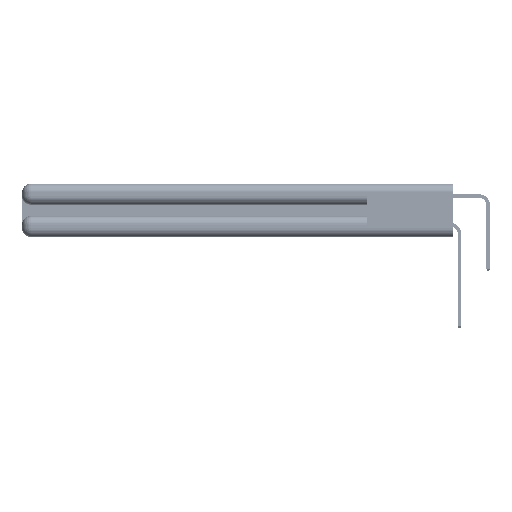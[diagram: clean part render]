
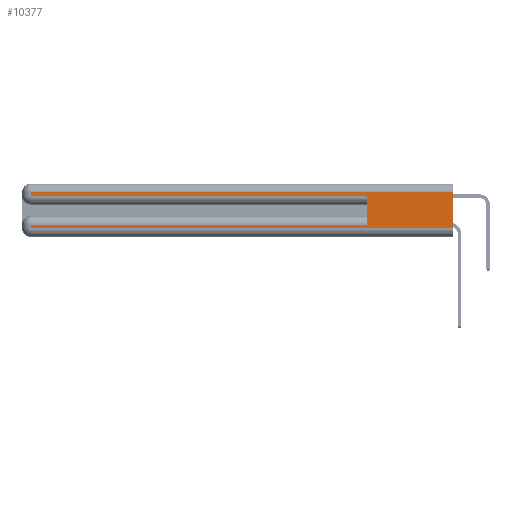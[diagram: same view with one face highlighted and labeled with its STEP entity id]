
A CAD part, left-side view. The second image highlights one B-rep face of the part: STEP entity #10377.
In plain terms, the highlighted planar face has unit normal (-1, 0, 0).
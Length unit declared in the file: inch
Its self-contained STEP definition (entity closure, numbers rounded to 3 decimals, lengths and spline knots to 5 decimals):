
#197 = CARTESIAN_POINT ( 'NONE',  ( 0., 0., 0.37 ) ) ;
#568 = DIRECTION ( 'NONE',  ( 1., 0., 0. ) ) ;
#743 = VECTOR ( 'NONE', #23854, 39.37008 ) ;
#811 = CARTESIAN_POINT ( 'NONE',  ( 0., 0.6, 0.085 ) ) ;
#1697 = ORIENTED_EDGE ( 'NONE', *, *, #26742, .T. ) ;
#2067 = CARTESIAN_POINT ( 'NONE',  ( 0., 0., 0.06 ) ) ;
#2609 = CARTESIAN_POINT ( 'NONE',  ( 0., 2.94, 0.06 ) ) ;
#2709 = LINE ( 'NONE', #13319, #29796 ) ;
#3090 = CARTESIAN_POINT ( 'NONE',  ( 0., 2.94, 0.285 ) ) ;
#3481 = EDGE_CURVE ( 'NONE', #26933, #31815, #48460, .T. ) ;
#3754 = DIRECTION ( 'NONE',  ( 0., 0., -1. ) ) ;
#5217 = VERTEX_POINT ( 'NONE', #19305 ) ;
#6022 = VERTEX_POINT ( 'NONE', #3090 ) ;
#6472 = VECTOR ( 'NONE', #3754, 39.37008 ) ;
#6734 = LINE ( 'NONE', #32748, #34508 ) ;
#7113 = LINE ( 'NONE', #20582, #6472 ) ;
#9104 = CARTESIAN_POINT ( 'NONE',  ( 0., 0., 0.37 ) ) ;
#10043 = LINE ( 'NONE', #11461, #743 ) ;
#10377 = ADVANCED_FACE ( 'NONE', ( #46119 ), #21132, .F. ) ;
#10402 = ORIENTED_EDGE ( 'NONE', *, *, #20596, .T. ) ;
#11461 = CARTESIAN_POINT ( 'NONE',  ( 0., 0., 0.06 ) ) ;
#12129 = EDGE_CURVE ( 'NONE', #44595, #35033, #36006, .T. ) ;
#12187 = LINE ( 'NONE', #9104, #54503 ) ;
#12201 = EDGE_CURVE ( 'NONE', #26933, #34320, #12187, .T. ) ;
#12446 = CARTESIAN_POINT ( 'NONE',  ( 0., 0., 0.31 ) ) ;
#13319 = CARTESIAN_POINT ( 'NONE',  ( 0., 0., 0.285 ) ) ;
#15855 = CARTESIAN_POINT ( 'NONE',  ( 0., 2.94, 0.37 ) ) ;
#17115 = VERTEX_POINT ( 'NONE', #2609 ) ;
#17213 = DIRECTION ( 'NONE',  ( 0., 0., -1. ) ) ;
#18166 = DIRECTION ( 'NONE',  ( 0., 0., 1. ) ) ;
#19305 = CARTESIAN_POINT ( 'NONE',  ( 0., 2.94, 0.085 ) ) ;
#20582 = CARTESIAN_POINT ( 'NONE',  ( 0., 2.94, 0.37 ) ) ;
#20596 = EDGE_CURVE ( 'NONE', #6022, #35033, #2709, .T. ) ;
#21132 = PLANE ( 'NONE',  #23270 ) ;
#22193 = ORIENTED_EDGE ( 'NONE', *, *, #54240, .T. ) ;
#22263 = EDGE_CURVE ( 'NONE', #31815, #6022, #7113, .T. ) ;
#23270 = AXIS2_PLACEMENT_3D ( 'NONE', #197, #568, #17213 ) ;
#23854 = DIRECTION ( 'NONE',  ( 0., -1., 0. ) ) ;
#24304 = EDGE_LOOP ( 'NONE', ( #32200, #50082, #53260, #10402, #26101, #1697, #24819, #22193 ) ) ;
#24819 = ORIENTED_EDGE ( 'NONE', *, *, #32434, .T. ) ;
#26101 = ORIENTED_EDGE ( 'NONE', *, *, #12129, .F. ) ;
#26742 = EDGE_CURVE ( 'NONE', #44595, #5217, #6734, .T. ) ;
#26933 = VERTEX_POINT ( 'NONE', #29251 ) ;
#27327 = CARTESIAN_POINT ( 'NONE',  ( 0., 0.6, 0.285 ) ) ;
#29251 = CARTESIAN_POINT ( 'NONE',  ( 0., 0., 0.31 ) ) ;
#29796 = VECTOR ( 'NONE', #51938, 39.37008 ) ;
#30705 = VECTOR ( 'NONE', #18166, 39.37008 ) ;
#31815 = VERTEX_POINT ( 'NONE', #44594 ) ;
#32200 = ORIENTED_EDGE ( 'NONE', *, *, #12201, .F. ) ;
#32434 = EDGE_CURVE ( 'NONE', #5217, #17115, #50234, .T. ) ;
#32675 = DIRECTION ( 'NONE',  ( 0., 0., -1. ) ) ;
#32748 = CARTESIAN_POINT ( 'NONE',  ( 0., 0., 0.085 ) ) ;
#34320 = VERTEX_POINT ( 'NONE', #2067 ) ;
#34508 = VECTOR ( 'NONE', #53638, 39.37008 ) ;
#34635 = DIRECTION ( 'NONE',  ( 0., 1., 0. ) ) ;
#35033 = VERTEX_POINT ( 'NONE', #27327 ) ;
#35911 = VECTOR ( 'NONE', #34635, 39.37008 ) ;
#36006 = LINE ( 'NONE', #38857, #30705 ) ;
#38676 = DIRECTION ( 'NONE',  ( 0., 0., -1. ) ) ;
#38857 = CARTESIAN_POINT ( 'NONE',  ( 0., 0.6, 0.145 ) ) ;
#44595 = VERTEX_POINT ( 'NONE', #811 ) ;
#44594 = CARTESIAN_POINT ( 'NONE',  ( 0., 2.94, 0.31 ) ) ;
#46119 = FACE_OUTER_BOUND ( 'NONE', #24304, .T. ) ;
#48460 = LINE ( 'NONE', #12446, #35911 ) ;
#50082 = ORIENTED_EDGE ( 'NONE', *, *, #3481, .T. ) ;
#50234 = LINE ( 'NONE', #15855, #53566 ) ;
#51938 = DIRECTION ( 'NONE',  ( 0., -1., 0. ) ) ;
#53260 = ORIENTED_EDGE ( 'NONE', *, *, #22263, .T. ) ;
#53566 = VECTOR ( 'NONE', #32675, 39.37008 ) ;
#53638 = DIRECTION ( 'NONE',  ( 0., 1., 0. ) ) ;
#54240 = EDGE_CURVE ( 'NONE', #17115, #34320, #10043, .T. ) ;
#54503 = VECTOR ( 'NONE', #38676, 39.37008 ) ;
